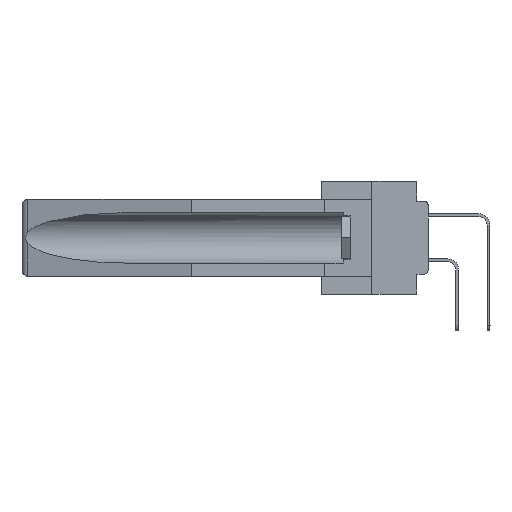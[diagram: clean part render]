
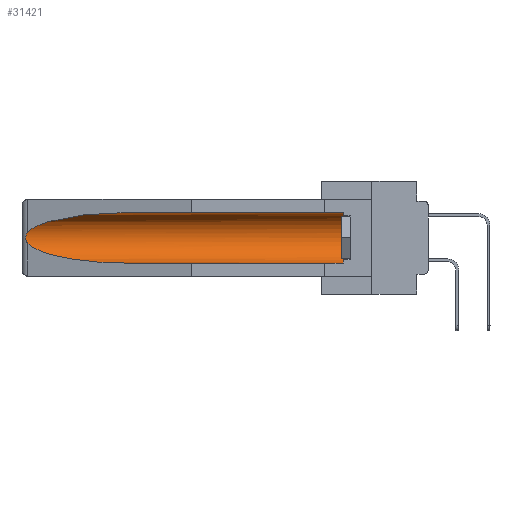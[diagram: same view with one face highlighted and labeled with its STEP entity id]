
A CAD part, left-side view. The second image highlights one B-rep face of the part: STEP entity #31421.
In plain terms, the highlighted cylindrical face has radius 2.857 mm (diameter 5.715 mm), a partial arc.
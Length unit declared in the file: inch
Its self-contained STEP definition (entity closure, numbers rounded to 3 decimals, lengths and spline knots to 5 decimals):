
#371 = VERTEX_POINT ( 'NONE', #39325 ) ;
#507 = DIRECTION ( 'NONE',  ( 0., -1., 0. ) ) ;
#1239 = DIRECTION ( 'NONE',  ( 0., 1., 0. ) ) ;
#2655 = CARTESIAN_POINT ( 'NONE',  ( 0.2675, 1.53308, -0.16763 ) ) ;
#2779 = CARTESIAN_POINT ( 'NONE',  ( 0.26655, 1.53094, -0.18657 ) ) ;
#3138 = CARTESIAN_POINT ( 'NONE',  ( 0.21114, 1.30732, -0.059 ) ) ;
#3913 = CARTESIAN_POINT ( 'NONE',  ( 0.155, 0.126, -0.1715 ) ) ;
#3916 = EDGE_CURVE ( 'NONE', #371, #18545, #32855, .T. ) ;
#5265 = VERTEX_POINT ( 'NONE', #8615 ) ;
#5313 = CARTESIAN_POINT ( 'NONE',  ( 0.26537, 1.52718, -0.14972 ) ) ;
#6067 = CARTESIAN_POINT ( 'NONE',  ( 0.25451, 1.48313, -0.24835 ) ) ;
#6500 = DIRECTION ( 'NONE',  ( 0., 1., 0. ) ) ;
#7852 = ORIENTED_EDGE ( 'NONE', *, *, #22575, .T. ) ;
#8615 = CARTESIAN_POINT ( 'NONE',  ( 0.26537, 1.52718, -0.19328 ) ) ;
#8932 = CARTESIAN_POINT ( 'NONE',  ( 0.2673, 1.53269, -0.17917 ) ) ;
#9058 = CARTESIAN_POINT ( 'NONE',  ( 0.2673, 1.5327, -0.16383 ) ) ;
#9183 = CARTESIAN_POINT ( 'NONE',  ( 0.2675, 1.53308, -0.17534 ) ) ;
#9481 = AXIS2_PLACEMENT_3D ( 'NONE', #32665, #1239, #16671 ) ;
#9488 = CARTESIAN_POINT ( 'NONE',  ( 0.155, -0.30754, -0.059 ) ) ;
#10279 = ORIENTED_EDGE ( 'NONE', *, *, #19865, .F. ) ;
#11931 = CARTESIAN_POINT ( 'NONE',  ( 0.26597, 1.5296, -0.19026 ) ) ;
#12088 = VERTEX_POINT ( 'NONE', #18238 ) ;
#12750 = DIRECTION ( 'NONE',  ( 0., 1., 0. ) ) ;
#12951 = FACE_OUTER_BOUND ( 'NONE', #23380, .T. ) ;
#13059 = CARTESIAN_POINT ( 'NONE',  ( 0.155, -0.30754, -0.284 ) ) ;
#15314 = VECTOR ( 'NONE', #6500, 39.37008 ) ;
#16440 =( BOUNDED_CURVE ( )  B_SPLINE_CURVE ( 3, ( #34125, #6067, #34511, #19428 ),
 .UNSPECIFIED., .F., .F. ) 
 B_SPLINE_CURVE_WITH_KNOTS ( ( 4, 4 ),
 ( 0.1948, 1.5708 ),
 .UNSPECIFIED. ) 
 CURVE ( )  GEOMETRIC_REPRESENTATION_ITEM ( )  RATIONAL_B_SPLINE_CURVE ( ( 1., 0.848, 0.848, 1. ) ) 
 REPRESENTATION_ITEM ( '' )  );
#16671 = DIRECTION ( 'NONE',  ( 0., 0., 1. ) ) ;
#17495 = EDGE_CURVE ( 'NONE', #19273, #5265, #19451, .T. ) ;
#17911 = CARTESIAN_POINT ( 'NONE',  ( 0.155, 0.126, -0.059 ) ) ;
#18238 = CARTESIAN_POINT ( 'NONE',  ( 0.155, 1.07973, -0.284 ) ) ;
#18545 = VERTEX_POINT ( 'NONE', #17911 ) ;
#18935 = VECTOR ( 'NONE', #12750, 39.37008 ) ;
#19037 = AXIS2_PLACEMENT_3D ( 'NONE', #3913, #507, #28926 ) ;
#19273 = VERTEX_POINT ( 'NONE', #19426 ) ;
#19426 = CARTESIAN_POINT ( 'NONE',  ( 0.26537, 1.52718, -0.14972 ) ) ;
#19428 = CARTESIAN_POINT ( 'NONE',  ( 0.155, 1.07973, -0.284 ) ) ;
#19451 = B_SPLINE_CURVE_WITH_KNOTS ( 'NONE', 3,
 ( #21474, #40366, #24363, #9058, #2655, #9183, #8932, #2779, #11931, #30776 ),
 .UNSPECIFIED., .F., .F.,
 ( 4, 2, 2, 2, 4 ),
 ( 0., 0.00029, 0.00058, 0.00087, 0.00117 ),
 .UNSPECIFIED. ) ;
#19865 = EDGE_CURVE ( 'NONE', #371, #12088, #29440, .T. ) ;
#21474 = CARTESIAN_POINT ( 'NONE',  ( 0.26537, 1.52718, -0.14972 ) ) ;
#22575 = EDGE_CURVE ( 'NONE', #18545, #34494, #37539, .T. ) ;
#23331 = ORIENTED_EDGE ( 'NONE', *, *, #31770, .T. ) ;
#23380 = EDGE_LOOP ( 'NONE', ( #23331, #25171, #38414, #10279, #38395, #7852 ) ) ;
#24363 = CARTESIAN_POINT ( 'NONE',  ( 0.26654, 1.53092, -0.15636 ) ) ;
#25171 = ORIENTED_EDGE ( 'NONE', *, *, #17495, .T. ) ;
#26106 = CARTESIAN_POINT ( 'NONE',  ( 0.25451, 1.48313, -0.09465 ) ) ;
#27131 =( BOUNDED_CURVE ( )  B_SPLINE_CURVE ( 3, ( #28149, #3138, #26106, #5313 ),
 .UNSPECIFIED., .F., .F. ) 
 B_SPLINE_CURVE_WITH_KNOTS ( ( 4, 4 ),
 ( 4.71239, 6.08839 ),
 .UNSPECIFIED. ) 
 CURVE ( )  GEOMETRIC_REPRESENTATION_ITEM ( )  RATIONAL_B_SPLINE_CURVE ( ( 1., 0.848, 0.848, 1. ) ) 
 REPRESENTATION_ITEM ( '' )  );
#28102 = CYLINDRICAL_SURFACE ( 'NONE', #9481, 0.1125 ) ;
#28149 = CARTESIAN_POINT ( 'NONE',  ( 0.155, 1.07973, -0.059 ) ) ;
#28483 = EDGE_CURVE ( 'NONE', #5265, #12088, #16440, .T. ) ;
#28926 = DIRECTION ( 'NONE',  ( 0., 0., 1. ) ) ;
#29440 = LINE ( 'NONE', #13059, #15314 ) ;
#30776 = CARTESIAN_POINT ( 'NONE',  ( 0.26537, 1.52718, -0.19328 ) ) ;
#31421 = ADVANCED_FACE ( 'NONE', ( #12951 ), #28102, .F. ) ;
#31770 = EDGE_CURVE ( 'NONE', #34494, #19273, #27131, .T. ) ;
#32093 = CARTESIAN_POINT ( 'NONE',  ( 0.155, 1.07973, -0.059 ) ) ;
#32665 = CARTESIAN_POINT ( 'NONE',  ( 0.155, -0.30754, -0.1715 ) ) ;
#32855 = CIRCLE ( 'NONE', #19037, 0.1125 ) ;
#34125 = CARTESIAN_POINT ( 'NONE',  ( 0.26537, 1.52718, -0.19328 ) ) ;
#34494 = VERTEX_POINT ( 'NONE', #32093 ) ;
#34511 = CARTESIAN_POINT ( 'NONE',  ( 0.21114, 1.30732, -0.284 ) ) ;
#37539 = LINE ( 'NONE', #9488, #18935 ) ;
#38395 = ORIENTED_EDGE ( 'NONE', *, *, #3916, .T. ) ;
#38414 = ORIENTED_EDGE ( 'NONE', *, *, #28483, .T. ) ;
#39325 = CARTESIAN_POINT ( 'NONE',  ( 0.155, 0.126, -0.284 ) ) ;
#40366 = CARTESIAN_POINT ( 'NONE',  ( 0.26597, 1.52961, -0.15275 ) ) ;
